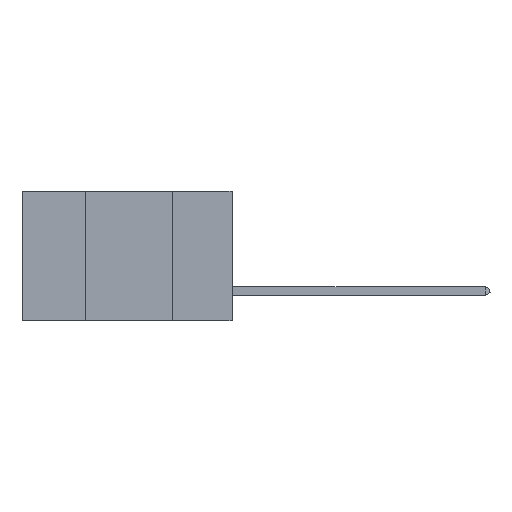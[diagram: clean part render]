
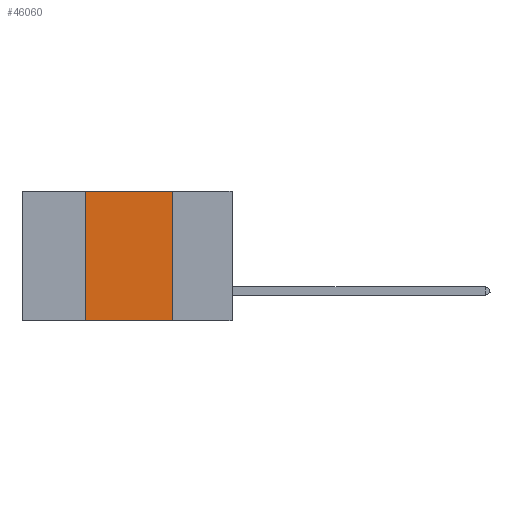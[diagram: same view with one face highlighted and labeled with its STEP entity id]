
A CAD part, left-side view. The second image highlights one B-rep face of the part: STEP entity #46060.
In plain terms, the highlighted planar face has unit normal (-1, 0, 0).
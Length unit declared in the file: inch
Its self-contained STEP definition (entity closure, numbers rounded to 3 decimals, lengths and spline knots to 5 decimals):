
#5702 = CARTESIAN_POINT ( 'NONE',  ( 0., 0.42, -0.37 ) ) ;
#7090 = VERTEX_POINT ( 'NONE', #5702 ) ;
#8042 = AXIS2_PLACEMENT_3D ( 'NONE', #10890, #30035, #18402 ) ;
#8713 = DIRECTION ( 'NONE',  ( 0., 0., 1. ) ) ;
#9928 = VECTOR ( 'NONE', #17208, 39.37008 ) ;
#10890 = CARTESIAN_POINT ( 'NONE',  ( 0., 0.6, 0. ) ) ;
#10999 = CARTESIAN_POINT ( 'NONE',  ( 0., 0.17, 0. ) ) ;
#14320 = EDGE_CURVE ( 'NONE', #29852, #39823, #28017, .T. ) ;
#14934 = CARTESIAN_POINT ( 'NONE',  ( 0., 0.42, 0. ) ) ;
#15493 = VECTOR ( 'NONE', #17716, 39.37008 ) ;
#15731 = VERTEX_POINT ( 'NONE', #14934 ) ;
#15881 = LINE ( 'NONE', #39604, #37886 ) ;
#17208 = DIRECTION ( 'NONE',  ( 0., -1., 0. ) ) ;
#17716 = DIRECTION ( 'NONE',  ( 0., 0., -1. ) ) ;
#17929 = DIRECTION ( 'NONE',  ( 0., -1., 0. ) ) ;
#18402 = DIRECTION ( 'NONE',  ( 0., 0., -1. ) ) ;
#22348 = ORIENTED_EDGE ( 'NONE', *, *, #43182, .F. ) ;
#24403 = CARTESIAN_POINT ( 'NONE',  ( 0., 0.6, -0.37 ) ) ;
#28017 = LINE ( 'NONE', #29678, #15493 ) ;
#29063 = CARTESIAN_POINT ( 'NONE',  ( 0., 0.6, 0. ) ) ;
#29678 = CARTESIAN_POINT ( 'NONE',  ( 0., 0.17, 0. ) ) ;
#29852 = VERTEX_POINT ( 'NONE', #10999 ) ;
#30035 = DIRECTION ( 'NONE',  ( 1., 0., 0. ) ) ;
#37401 = PLANE ( 'NONE',  #8042 ) ;
#37886 = VECTOR ( 'NONE', #8713, 39.37008 ) ;
#39604 = CARTESIAN_POINT ( 'NONE',  ( 0., 0.42, 0. ) ) ;
#39786 = LINE ( 'NONE', #24403, #9928 ) ;
#39823 = VERTEX_POINT ( 'NONE', #43382 ) ;
#39981 = ORIENTED_EDGE ( 'NONE', *, *, #14320, .F. ) ;
#41557 = EDGE_LOOP ( 'NONE', ( #39981, #47308, #22348, #46771 ) ) ;
#41910 = LINE ( 'NONE', #29063, #45486 ) ;
#42459 = EDGE_CURVE ( 'NONE', #7090, #39823, #39786, .T. ) ;
#43041 = FACE_OUTER_BOUND ( 'NONE', #41557, .T. ) ;
#43182 = EDGE_CURVE ( 'NONE', #7090, #15731, #15881, .T. ) ;
#43382 = CARTESIAN_POINT ( 'NONE',  ( 0., 0.17, -0.37 ) ) ;
#45486 = VECTOR ( 'NONE', #17929, 39.37008 ) ;
#45812 = EDGE_CURVE ( 'NONE', #15731, #29852, #41910, .T. ) ;
#46060 = ADVANCED_FACE ( 'NONE', ( #43041 ), #37401, .F. ) ;
#46771 = ORIENTED_EDGE ( 'NONE', *, *, #42459, .T. ) ;
#47308 = ORIENTED_EDGE ( 'NONE', *, *, #45812, .F. ) ;
